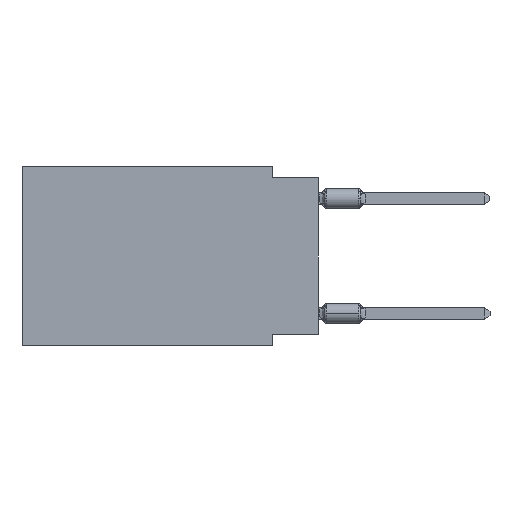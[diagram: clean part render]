
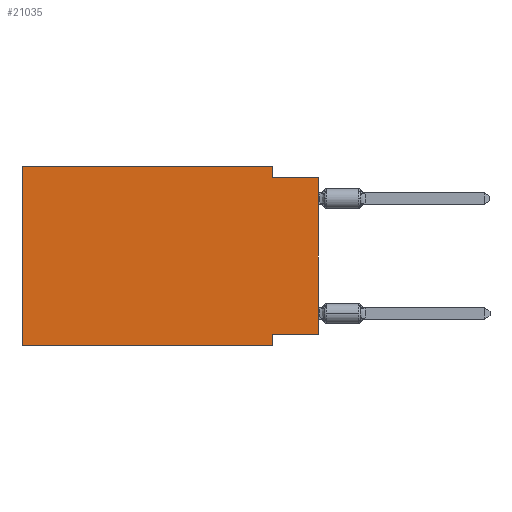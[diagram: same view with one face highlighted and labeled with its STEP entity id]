
A CAD part, left-side view. The second image highlights one B-rep face of the part: STEP entity #21035.
In plain terms, the highlighted planar face has unit normal (-1, 0, 0).
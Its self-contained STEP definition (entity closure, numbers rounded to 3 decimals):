
#727 = VECTOR ( 'NONE', #17997, 1000. ) ;
#927 = CARTESIAN_POINT ( 'NONE',  ( 0., 2.54, -9.271 ) ) ;
#2668 = CARTESIAN_POINT ( 'NONE',  ( 0., 2.54, 0. ) ) ;
#2788 = CARTESIAN_POINT ( 'NONE',  ( 0., 2.54, -9.906 ) ) ;
#2984 = EDGE_CURVE ( 'NONE', #18044, #14367, #17899, .T. ) ;
#3013 = LINE ( 'NONE', #2788, #20915 ) ;
#3429 = CARTESIAN_POINT ( 'NONE',  ( 0., 16.383, 0. ) ) ;
#3492 = CARTESIAN_POINT ( 'NONE',  ( 0., 2.54, -9.906 ) ) ;
#4398 = ORIENTED_EDGE ( 'NONE', *, *, #16850, .F. ) ;
#4895 = VECTOR ( 'NONE', #13357, 1000. ) ;
#4972 = VECTOR ( 'NONE', #16193, 1000. ) ;
#5088 = LINE ( 'NONE', #8347, #727 ) ;
#5795 = ORIENTED_EDGE ( 'NONE', *, *, #19729, .F. ) ;
#5826 = DIRECTION ( 'NONE',  ( 0., -1., 0. ) ) ;
#6097 = LINE ( 'NONE', #12726, #12931 ) ;
#7482 = ORIENTED_EDGE ( 'NONE', *, *, #16456, .F. ) ;
#7953 = EDGE_CURVE ( 'NONE', #16569, #14367, #12358, .T. ) ;
#8228 = ORIENTED_EDGE ( 'NONE', *, *, #17707, .F. ) ;
#8292 = PLANE ( 'NONE',  #12272 ) ;
#8347 = CARTESIAN_POINT ( 'NONE',  ( 0., 16.383, -9.906 ) ) ;
#8547 = EDGE_LOOP ( 'NONE', ( #13566, #16654, #7482, #4398, #5795, #15915, #8228, #12652 ) ) ;
#8558 = VERTEX_POINT ( 'NONE', #3492 ) ;
#9153 = CARTESIAN_POINT ( 'NONE',  ( 0., 0., -9.271 ) ) ;
#9614 = VERTEX_POINT ( 'NONE', #2668 ) ;
#11040 = CARTESIAN_POINT ( 'NONE',  ( 0., 0., -9.271 ) ) ;
#11354 = EDGE_CURVE ( 'NONE', #14077, #8558, #5088, .T. ) ;
#11782 = VECTOR ( 'NONE', #18079, 1000. ) ;
#11831 = VECTOR ( 'NONE', #5826, 1000. ) ;
#12169 = EDGE_CURVE ( 'NONE', #18044, #15675, #16037, .T. ) ;
#12272 = AXIS2_PLACEMENT_3D ( 'NONE', #3429, #13508, #18267 ) ;
#12358 = LINE ( 'NONE', #15813, #11831 ) ;
#12433 = CARTESIAN_POINT ( 'NONE',  ( 0., 2.54, 0. ) ) ;
#12528 = CARTESIAN_POINT ( 'NONE',  ( 0., 16.383, 0. ) ) ;
#12652 = ORIENTED_EDGE ( 'NONE', *, *, #12169, .F. ) ;
#12726 = CARTESIAN_POINT ( 'NONE',  ( 0., 16.383, 0. ) ) ;
#12931 = VECTOR ( 'NONE', #19309, 1000. ) ;
#12990 = DIRECTION ( 'NONE',  ( 0., 0., -1. ) ) ;
#13067 = LINE ( 'NONE', #12433, #4972 ) ;
#13357 = DIRECTION ( 'NONE',  ( 0., 0., 1. ) ) ;
#13508 = DIRECTION ( 'NONE',  ( 1., 0., 0. ) ) ;
#13566 = ORIENTED_EDGE ( 'NONE', *, *, #2984, .T. ) ;
#14077 = VERTEX_POINT ( 'NONE', #15353 ) ;
#14367 = VERTEX_POINT ( 'NONE', #18143 ) ;
#15238 = FACE_OUTER_BOUND ( 'NONE', #8547, .T. ) ;
#15353 = CARTESIAN_POINT ( 'NONE',  ( 0., 16.383, -9.906 ) ) ;
#15675 = VERTEX_POINT ( 'NONE', #927 ) ;
#15813 = CARTESIAN_POINT ( 'NONE',  ( 0., 0., -0.635 ) ) ;
#15915 = ORIENTED_EDGE ( 'NONE', *, *, #11354, .T. ) ;
#16037 = LINE ( 'NONE', #11040, #11782 ) ;
#16085 = VECTOR ( 'NONE', #21018, 1000. ) ;
#16193 = DIRECTION ( 'NONE',  ( 0., 0., -1. ) ) ;
#16456 = EDGE_CURVE ( 'NONE', #9614, #16569, #13067, .T. ) ;
#16569 = VERTEX_POINT ( 'NONE', #18646 ) ;
#16654 = ORIENTED_EDGE ( 'NONE', *, *, #7953, .F. ) ;
#16850 = EDGE_CURVE ( 'NONE', #19284, #9614, #21124, .T. ) ;
#17707 = EDGE_CURVE ( 'NONE', #15675, #8558, #3013, .T. ) ;
#17899 = LINE ( 'NONE', #18103, #4895 ) ;
#17997 = DIRECTION ( 'NONE',  ( 0., -1., 0. ) ) ;
#18044 = VERTEX_POINT ( 'NONE', #9153 ) ;
#18079 = DIRECTION ( 'NONE',  ( 0., 1., 0. ) ) ;
#18103 = CARTESIAN_POINT ( 'NONE',  ( 0., 0., 0. ) ) ;
#18143 = CARTESIAN_POINT ( 'NONE',  ( 0., 0., -0.635 ) ) ;
#18267 = DIRECTION ( 'NONE',  ( 0., 0., -1. ) ) ;
#18646 = CARTESIAN_POINT ( 'NONE',  ( 0., 2.54, -0.635 ) ) ;
#19284 = VERTEX_POINT ( 'NONE', #12528 ) ;
#19309 = DIRECTION ( 'NONE',  ( 0., 0., 1. ) ) ;
#19621 = CARTESIAN_POINT ( 'NONE',  ( 0., 16.383, 0. ) ) ;
#19729 = EDGE_CURVE ( 'NONE', #14077, #19284, #6097, .T. ) ;
#20915 = VECTOR ( 'NONE', #12990, 1000. ) ;
#21018 = DIRECTION ( 'NONE',  ( 0., -1., 0. ) ) ;
#21035 = ADVANCED_FACE ( 'NONE', ( #15238 ), #8292, .F. ) ;
#21124 = LINE ( 'NONE', #19621, #16085 ) ;
